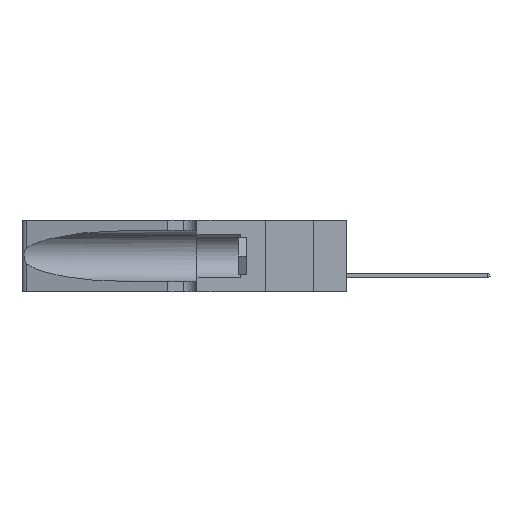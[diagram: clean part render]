
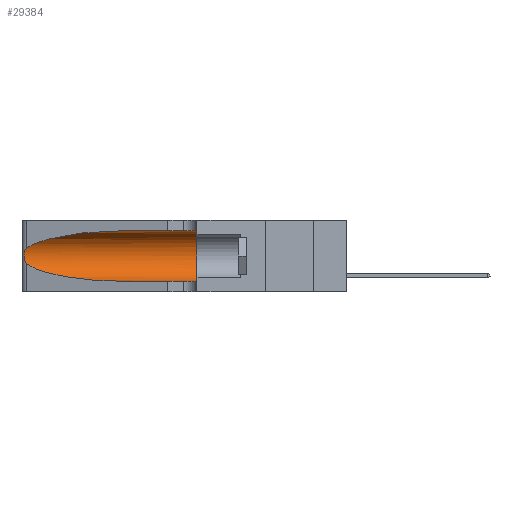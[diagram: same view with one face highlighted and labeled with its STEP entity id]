
A CAD part, left-side view. The second image highlights one B-rep face of the part: STEP entity #29384.
In plain terms, the highlighted cylindrical face has radius 3.308 mm (diameter 6.617 mm), a partial arc.
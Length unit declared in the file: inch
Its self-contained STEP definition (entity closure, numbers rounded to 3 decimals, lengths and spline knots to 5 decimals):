
#924 = LINE ( 'NONE', #23505, #23844 ) ;
#1393 = CARTESIAN_POINT ( 'NONE',  ( 0.25487, 1.22718, 0.22369 ) ) ;
#1740 = VERTEX_POINT ( 'NONE', #26925 ) ;
#2829 = ORIENTED_EDGE ( 'NONE', *, *, #4025, .F. ) ;
#3236 = VERTEX_POINT ( 'NONE', #3572 ) ;
#3572 = CARTESIAN_POINT ( 'NONE',  ( 0.1305, 0.72297, 0.05475 ) ) ;
#4025 = EDGE_CURVE ( 'NONE', #16432, #16755, #17995, .T. ) ;
#4220 = DIRECTION ( 'NONE',  ( 0., 0., 1. ) ) ;
#5678 = EDGE_CURVE ( 'NONE', #3236, #16755, #924, .T. ) ;
#5776 = CARTESIAN_POINT ( 'NONE',  ( 0.2373, 1.15595, 0.08982 ) ) ;
#5882 = CARTESIAN_POINT ( 'NONE',  ( 0.25487, 1.22718, 0.14631 ) ) ;
#6240 = CARTESIAN_POINT ( 'NONE',  ( 0.25487, 1.22718, 0.22369 ) ) ;
#6583 = CARTESIAN_POINT ( 'NONE',  ( 0.1305, 0.35, 0.185 ) ) ;
#7716 = EDGE_CURVE ( 'NONE', #30214, #16432, #13771, .T. ) ;
#9159 = AXIS2_PLACEMENT_3D ( 'NONE', #29072, #16268, #29182 ) ;
#9376 = VECTOR ( 'NONE', #32154, 39.37008 ) ;
#11435 = CARTESIAN_POINT ( 'NONE',  ( 0.26075, 1.23896, 0.178 ) ) ;
#11993 = CARTESIAN_POINT ( 'NONE',  ( 0.25856, 1.23593, 0.16098 ) ) ;
#12120 = CARTESIAN_POINT ( 'NONE',  ( 0.25487, 1.22718, 0.14631 ) ) ;
#12457 = CARTESIAN_POINT ( 'NONE',  ( 0.25555, 1.22993, 0.14849 ) ) ;
#12692 = EDGE_CURVE ( 'NONE', #30214, #30147, #18890, .T. ) ;
#13771 = LINE ( 'NONE', #24498, #9376 ) ;
#14124 = CARTESIAN_POINT ( 'NONE',  ( 0.25639, 1.23184, 0.21858 ) ) ;
#14698 = CARTESIAN_POINT ( 'NONE',  ( 0.25639, 1.23186, 0.15144 ) ) ;
#15696 = DIRECTION ( 'NONE',  ( 0., -1., 0. ) ) ;
#16147 = CARTESIAN_POINT ( 'NONE',  ( 0.18966, 0.96281, 0.31525 ) ) ;
#16268 = DIRECTION ( 'NONE',  ( 0., -1., 0. ) ) ;
#16432 = VERTEX_POINT ( 'NONE', #27677 ) ;
#16462 = B_SPLINE_CURVE_WITH_KNOTS ( 'NONE', 3,
 ( #1393, #19470, #14124, #31965, #22166, #24192, #26815, #11435, #27633, #11993, #19694, #14698, #12457, #12120 ),
 .UNSPECIFIED., .F., .F.,
 ( 4, 2, 2, 2, 2, 2, 4 ),
 ( 0., 0.00027, 0.00053, 0.00107, 0.0016, 0.00187, 0.00214 ),
 .UNSPECIFIED. ) ;
#16755 = VERTEX_POINT ( 'NONE', #18117 ) ;
#16776 = AXIS2_PLACEMENT_3D ( 'NONE', #6583, #16951, #4220 ) ;
#16951 = DIRECTION ( 'NONE',  ( 0., 1., 0. ) ) ;
#17995 = CIRCLE ( 'NONE', #16776, 0.13025 ) ;
#18117 = CARTESIAN_POINT ( 'NONE',  ( 0.1305, 0.35, 0.05475 ) ) ;
#18316 = CARTESIAN_POINT ( 'NONE',  ( 0.25487, 1.22718, 0.22369 ) ) ;
#18890 =( BOUNDED_CURVE ( )  B_SPLINE_CURVE ( 3, ( #20437, #16147, #23951, #6240 ),
 .UNSPECIFIED., .F., .F. ) 
 B_SPLINE_CURVE_WITH_KNOTS ( ( 4, 4 ),
 ( 1.5708, 2.84003 ),
 .UNSPECIFIED. ) 
 CURVE ( )  GEOMETRIC_REPRESENTATION_ITEM ( )  RATIONAL_B_SPLINE_CURVE ( ( 1., 0.87, 0.87, 1. ) ) 
 REPRESENTATION_ITEM ( '' )  );
#19470 = CARTESIAN_POINT ( 'NONE',  ( 0.25555, 1.22994, 0.2215 ) ) ;
#19694 = CARTESIAN_POINT ( 'NONE',  ( 0.25789, 1.23486, 0.15765 ) ) ;
#19706 = ORIENTED_EDGE ( 'NONE', *, *, #7716, .F. ) ;
#20215 = ORIENTED_EDGE ( 'NONE', *, *, #12692, .T. ) ;
#20243 = ORIENTED_EDGE ( 'NONE', *, *, #21173, .T. ) ;
#20437 = CARTESIAN_POINT ( 'NONE',  ( 0.1305, 0.72297, 0.31525 ) ) ;
#21173 = EDGE_CURVE ( 'NONE', #1740, #3236, #31909, .T. ) ;
#21921 = EDGE_LOOP ( 'NONE', ( #20215, #31457, #20243, #23868, #2829, #19706 ) ) ;
#22166 = CARTESIAN_POINT ( 'NONE',  ( 0.25854, 1.2359, 0.20912 ) ) ;
#22234 = FACE_OUTER_BOUND ( 'NONE', #21921, .T. ) ;
#23505 = CARTESIAN_POINT ( 'NONE',  ( 0.1305, 1.61858, 0.05475 ) ) ;
#23738 = CARTESIAN_POINT ( 'NONE',  ( 0.18966, 0.96281, 0.05475 ) ) ;
#23844 = VECTOR ( 'NONE', #15696, 39.37008 ) ;
#23861 = CARTESIAN_POINT ( 'NONE',  ( 0.1305, 0.72297, 0.05475 ) ) ;
#23868 = ORIENTED_EDGE ( 'NONE', *, *, #5678, .T. ) ;
#23951 = CARTESIAN_POINT ( 'NONE',  ( 0.2373, 1.15595, 0.28018 ) ) ;
#24192 = CARTESIAN_POINT ( 'NONE',  ( 0.26018, 1.23835, 0.19895 ) ) ;
#24498 = CARTESIAN_POINT ( 'NONE',  ( 0.1305, 1.61858, 0.31525 ) ) ;
#25068 = CYLINDRICAL_SURFACE ( 'NONE', #9159, 0.13025 ) ;
#26218 = CARTESIAN_POINT ( 'NONE',  ( 0.1305, 0.72297, 0.31525 ) ) ;
#26815 = CARTESIAN_POINT ( 'NONE',  ( 0.26075, 1.23896, 0.19203 ) ) ;
#26925 = CARTESIAN_POINT ( 'NONE',  ( 0.25487, 1.22718, 0.14631 ) ) ;
#27633 = CARTESIAN_POINT ( 'NONE',  ( 0.26017, 1.23833, 0.17102 ) ) ;
#27677 = CARTESIAN_POINT ( 'NONE',  ( 0.1305, 0.35, 0.31525 ) ) ;
#29072 = CARTESIAN_POINT ( 'NONE',  ( 0.1305, 1.61858, 0.185 ) ) ;
#29182 = DIRECTION ( 'NONE',  ( 0., 0., -1. ) ) ;
#29384 = ADVANCED_FACE ( 'NONE', ( #22234 ), #25068, .F. ) ;
#30147 = VERTEX_POINT ( 'NONE', #18316 ) ;
#30214 = VERTEX_POINT ( 'NONE', #26218 ) ;
#31457 = ORIENTED_EDGE ( 'NONE', *, *, #32026, .T. ) ;
#31909 =( BOUNDED_CURVE ( )  B_SPLINE_CURVE ( 3, ( #5882, #5776, #23738, #23861 ),
 .UNSPECIFIED., .F., .F. ) 
 B_SPLINE_CURVE_WITH_KNOTS ( ( 4, 4 ),
 ( 3.44316, 4.71239 ),
 .UNSPECIFIED. ) 
 CURVE ( )  GEOMETRIC_REPRESENTATION_ITEM ( )  RATIONAL_B_SPLINE_CURVE ( ( 1., 0.87, 0.87, 1. ) ) 
 REPRESENTATION_ITEM ( '' )  );
#31965 = CARTESIAN_POINT ( 'NONE',  ( 0.25787, 1.23484, 0.2124 ) ) ;
#32026 = EDGE_CURVE ( 'NONE', #30147, #1740, #16462, .T. ) ;
#32154 = DIRECTION ( 'NONE',  ( 0., -1., 0. ) ) ;
